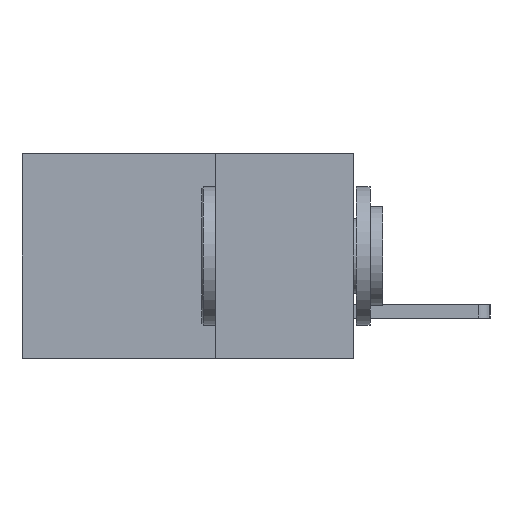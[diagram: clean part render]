
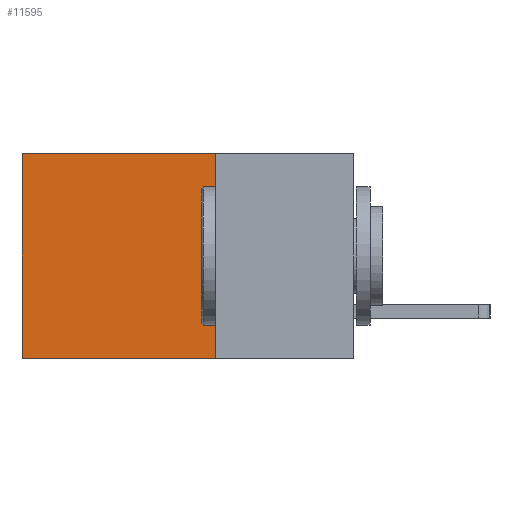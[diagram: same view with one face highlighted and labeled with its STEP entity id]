
A CAD part, left-side view. The second image highlights one B-rep face of the part: STEP entity #11595.
In plain terms, the highlighted planar face has unit normal (-1, 0, 0).
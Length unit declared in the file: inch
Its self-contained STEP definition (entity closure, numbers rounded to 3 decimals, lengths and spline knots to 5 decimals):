
#443 = LINE ( 'NONE', #9078, #1054 ) ;
#529 = EDGE_CURVE ( 'NONE', #8380, #6013, #10448, .T. ) ;
#968 = VECTOR ( 'NONE', #12997, 39.37008 ) ;
#1054 = VECTOR ( 'NONE', #12104, 39.37008 ) ;
#1219 = CARTESIAN_POINT ( 'NONE',  ( 0.2875, 0.6, 0. ) ) ;
#1563 = CARTESIAN_POINT ( 'NONE',  ( 0.2875, 0.6, 0. ) ) ;
#3284 = DIRECTION ( 'NONE',  ( 0., 0., -1. ) ) ;
#3563 = ORIENTED_EDGE ( 'NONE', *, *, #11721, .T. ) ;
#3857 = VECTOR ( 'NONE', #11480, 39.37008 ) ;
#3965 = FACE_OUTER_BOUND ( 'NONE', #12880, .T. ) ;
#4592 = CARTESIAN_POINT ( 'NONE',  ( 0.2875, 0.25, -0.37 ) ) ;
#4738 = VERTEX_POINT ( 'NONE', #1219 ) ;
#6013 = VERTEX_POINT ( 'NONE', #6858 ) ;
#6740 = VECTOR ( 'NONE', #3284, 39.37008 ) ;
#6858 = CARTESIAN_POINT ( 'NONE',  ( 0.2875, 0.6, -0.37 ) ) ;
#7106 = ORIENTED_EDGE ( 'NONE', *, *, #13171, .T. ) ;
#7539 = DIRECTION ( 'NONE',  ( 1., 0., 0. ) ) ;
#8027 = VERTEX_POINT ( 'NONE', #10507 ) ;
#8172 = CARTESIAN_POINT ( 'NONE',  ( 0.2875, 0.25, 0. ) ) ;
#8252 = PLANE ( 'NONE',  #8511 ) ;
#8380 = VERTEX_POINT ( 'NONE', #4592 ) ;
#8469 = CARTESIAN_POINT ( 'NONE',  ( 0.2875, 0.25, -0.37 ) ) ;
#8511 = AXIS2_PLACEMENT_3D ( 'NONE', #8172, #7539, #10637 ) ;
#9078 = CARTESIAN_POINT ( 'NONE',  ( 0.2875, 0.25, 0. ) ) ;
#9670 = LINE ( 'NONE', #10824, #6740 ) ;
#10448 = LINE ( 'NONE', #8469, #3857 ) ;
#10507 = CARTESIAN_POINT ( 'NONE',  ( 0.2875, 0.25, 0. ) ) ;
#10637 = DIRECTION ( 'NONE',  ( 0., 0., -1. ) ) ;
#10779 = ORIENTED_EDGE ( 'NONE', *, *, #529, .F. ) ;
#10824 = CARTESIAN_POINT ( 'NONE',  ( 0.2875, 0.25, 0. ) ) ;
#11034 = LINE ( 'NONE', #1563, #968 ) ;
#11480 = DIRECTION ( 'NONE',  ( 0., 1., 0. ) ) ;
#11595 = ADVANCED_FACE ( 'NONE', ( #3965 ), #8252, .F. ) ;
#11721 = EDGE_CURVE ( 'NONE', #4738, #6013, #11034, .T. ) ;
#12080 = ORIENTED_EDGE ( 'NONE', *, *, #12169, .F. ) ;
#12104 = DIRECTION ( 'NONE',  ( 0., 1., 0. ) ) ;
#12169 = EDGE_CURVE ( 'NONE', #8027, #8380, #9670, .T. ) ;
#12880 = EDGE_LOOP ( 'NONE', ( #3563, #10779, #12080, #7106 ) ) ;
#12997 = DIRECTION ( 'NONE',  ( 0., 0., -1. ) ) ;
#13171 = EDGE_CURVE ( 'NONE', #8027, #4738, #443, .T. ) ;
